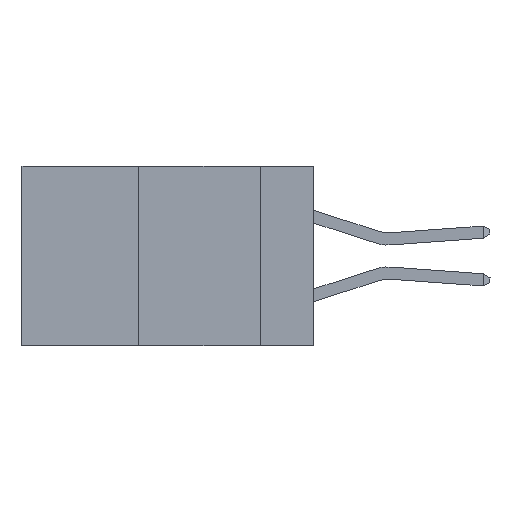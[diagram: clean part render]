
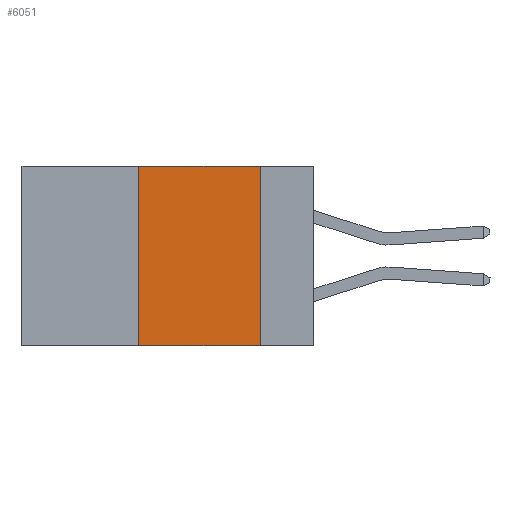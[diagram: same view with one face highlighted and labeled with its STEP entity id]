
A CAD part, left-side view. The second image highlights one B-rep face of the part: STEP entity #6051.
In plain terms, the highlighted planar face has unit normal (-1, 0, 0).
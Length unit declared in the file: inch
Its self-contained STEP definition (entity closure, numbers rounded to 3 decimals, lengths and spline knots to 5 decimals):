
#1641 = DIRECTION ( 'NONE',  ( 0., -1., 0. ) ) ;
#1645 = VERTEX_POINT ( 'NONE', #6357 ) ;
#1877 = CARTESIAN_POINT ( 'NONE',  ( 0., 0.6, 0. ) ) ;
#2908 = EDGE_CURVE ( 'NONE', #7310, #1645, #6277, .T. ) ;
#2996 = DIRECTION ( 'NONE',  ( 0., -1., 0. ) ) ;
#3030 = CARTESIAN_POINT ( 'NONE',  ( 0., 0.36, -0.37 ) ) ;
#3115 = CARTESIAN_POINT ( 'NONE',  ( 0., 0.36, 0. ) ) ;
#4363 = CARTESIAN_POINT ( 'NONE',  ( 0., 0.36, 0. ) ) ;
#4480 = LINE ( 'NONE', #5290, #7126 ) ;
#5081 = FACE_OUTER_BOUND ( 'NONE', #7551, .T. ) ;
#5290 = CARTESIAN_POINT ( 'NONE',  ( 0., 0.11, 0. ) ) ;
#6051 = ADVANCED_FACE ( 'NONE', ( #5081 ), #8877, .F. ) ;
#6277 = LINE ( 'NONE', #1877, #9307 ) ;
#6336 = DIRECTION ( 'NONE',  ( 0., 0., -1. ) ) ;
#6357 = CARTESIAN_POINT ( 'NONE',  ( 0., 0.11, 0. ) ) ;
#6928 = CARTESIAN_POINT ( 'NONE',  ( 0., 0.6, -0.37 ) ) ;
#7126 = VECTOR ( 'NONE', #10442, 39.37008 ) ;
#7310 = VERTEX_POINT ( 'NONE', #3115 ) ;
#7495 = LINE ( 'NONE', #4363, #13844 ) ;
#7551 = EDGE_LOOP ( 'NONE', ( #13059, #16348, #16731, #14999 ) ) ;
#8625 = VECTOR ( 'NONE', #2996, 39.37008 ) ;
#8877 = PLANE ( 'NONE',  #15361 ) ;
#9307 = VECTOR ( 'NONE', #1641, 39.37008 ) ;
#9548 = CARTESIAN_POINT ( 'NONE',  ( 0., 0.11, -0.37 ) ) ;
#9563 = DIRECTION ( 'NONE',  ( 0., 0., 1. ) ) ;
#9656 = VERTEX_POINT ( 'NONE', #9548 ) ;
#10130 = EDGE_CURVE ( 'NONE', #1645, #9656, #4480, .T. ) ;
#10442 = DIRECTION ( 'NONE',  ( 0., 0., -1. ) ) ;
#10987 = EDGE_CURVE ( 'NONE', #12451, #7310, #7495, .T. ) ;
#12029 = LINE ( 'NONE', #6928, #8625 ) ;
#12451 = VERTEX_POINT ( 'NONE', #3030 ) ;
#12726 = CARTESIAN_POINT ( 'NONE',  ( 0., 0.6, 0. ) ) ;
#13059 = ORIENTED_EDGE ( 'NONE', *, *, #10130, .F. ) ;
#13510 = EDGE_CURVE ( 'NONE', #12451, #9656, #12029, .T. ) ;
#13844 = VECTOR ( 'NONE', #9563, 39.37008 ) ;
#13944 = DIRECTION ( 'NONE',  ( 1., 0., 0. ) ) ;
#14999 = ORIENTED_EDGE ( 'NONE', *, *, #13510, .T. ) ;
#15361 = AXIS2_PLACEMENT_3D ( 'NONE', #12726, #13944, #6336 ) ;
#16348 = ORIENTED_EDGE ( 'NONE', *, *, #2908, .F. ) ;
#16731 = ORIENTED_EDGE ( 'NONE', *, *, #10987, .F. ) ;
